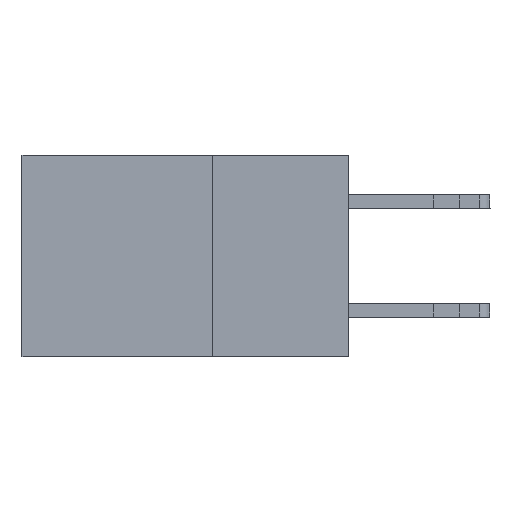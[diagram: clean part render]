
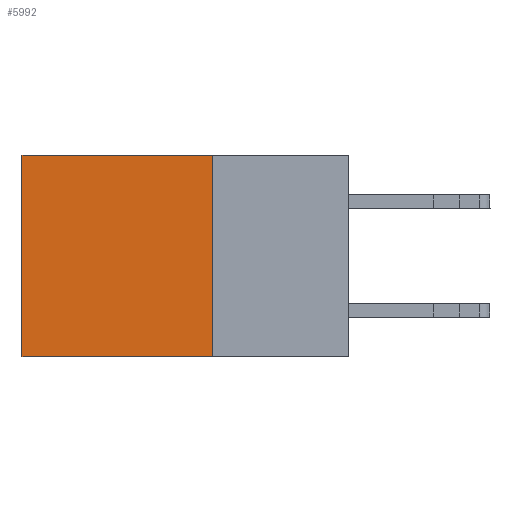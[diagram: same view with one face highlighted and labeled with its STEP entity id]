
A CAD part, left-side view. The second image highlights one B-rep face of the part: STEP entity #5992.
In plain terms, the highlighted planar face has unit normal (-1, 0, 0).
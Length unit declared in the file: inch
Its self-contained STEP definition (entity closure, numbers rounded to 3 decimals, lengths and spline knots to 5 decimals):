
#202 = CARTESIAN_POINT ( 'NONE',  ( 0.2615, 0.25, -0.37 ) ) ;
#528 = AXIS2_PLACEMENT_3D ( 'NONE', #202, #16113, #1906 ) ;
#1036 = DIRECTION ( 'NONE',  ( 0., 0., -1. ) ) ;
#1694 = ORIENTED_EDGE ( 'NONE', *, *, #14080, .F. ) ;
#1906 = DIRECTION ( 'NONE',  ( 0., 0., -1. ) ) ;
#2497 = CARTESIAN_POINT ( 'NONE',  ( 0.2615, 0.6, -0.37 ) ) ;
#3345 = LINE ( 'NONE', #13101, #18756 ) ;
#3449 = DIRECTION ( 'NONE',  ( 0., 1., 0. ) ) ;
#3455 = DIRECTION ( 'NONE',  ( 0., 0., -1. ) ) ;
#5142 = EDGE_CURVE ( 'NONE', #6826, #11909, #3345, .T. ) ;
#5597 = CARTESIAN_POINT ( 'NONE',  ( 0.2615, 0.25, -0.37 ) ) ;
#5992 = ADVANCED_FACE ( 'NONE', ( #11667 ), #18107, .F. ) ;
#6664 = VECTOR ( 'NONE', #18256, 39.37008 ) ;
#6826 = VERTEX_POINT ( 'NONE', #19310 ) ;
#7816 = ORIENTED_EDGE ( 'NONE', *, *, #20174, .F. ) ;
#8096 = VERTEX_POINT ( 'NONE', #17550 ) ;
#9087 = LINE ( 'NONE', #5597, #14587 ) ;
#10130 = LINE ( 'NONE', #17962, #11717 ) ;
#10925 = EDGE_CURVE ( 'NONE', #13120, #6826, #10130, .T. ) ;
#11470 = CARTESIAN_POINT ( 'NONE',  ( 0.2615, 0.25, 0. ) ) ;
#11667 = FACE_OUTER_BOUND ( 'NONE', #12554, .T. ) ;
#11717 = VECTOR ( 'NONE', #3449, 39.37008 ) ;
#11809 = CARTESIAN_POINT ( 'NONE',  ( 0.2615, 0.25, -0.37 ) ) ;
#11909 = VERTEX_POINT ( 'NONE', #2497 ) ;
#12554 = EDGE_LOOP ( 'NONE', ( #19614, #1694, #7816, #14531 ) ) ;
#13101 = CARTESIAN_POINT ( 'NONE',  ( 0.2615, 0.6, -0.37 ) ) ;
#13120 = VERTEX_POINT ( 'NONE', #11470 ) ;
#13391 = LINE ( 'NONE', #11809, #6664 ) ;
#14080 = EDGE_CURVE ( 'NONE', #8096, #11909, #13391, .T. ) ;
#14531 = ORIENTED_EDGE ( 'NONE', *, *, #10925, .T. ) ;
#14587 = VECTOR ( 'NONE', #1036, 39.37008 ) ;
#16113 = DIRECTION ( 'NONE',  ( 1., 0., 0. ) ) ;
#17550 = CARTESIAN_POINT ( 'NONE',  ( 0.2615, 0.25, -0.37 ) ) ;
#17962 = CARTESIAN_POINT ( 'NONE',  ( 0.2615, 0.25, 0. ) ) ;
#18107 = PLANE ( 'NONE',  #528 ) ;
#18256 = DIRECTION ( 'NONE',  ( 0., 1., 0. ) ) ;
#18756 = VECTOR ( 'NONE', #3455, 39.37008 ) ;
#19310 = CARTESIAN_POINT ( 'NONE',  ( 0.2615, 0.6, 0. ) ) ;
#19614 = ORIENTED_EDGE ( 'NONE', *, *, #5142, .T. ) ;
#20174 = EDGE_CURVE ( 'NONE', #13120, #8096, #9087, .T. ) ;
